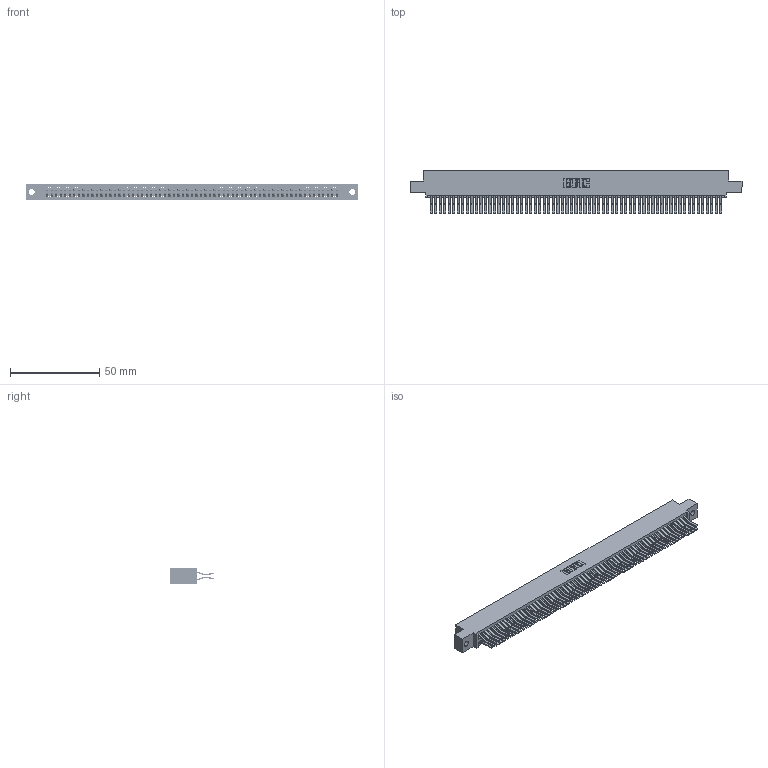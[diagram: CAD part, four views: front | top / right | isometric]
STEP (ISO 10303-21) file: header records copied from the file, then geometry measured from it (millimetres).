
FILE_DESCRIPTION (( 'STEP AP203' ), '1' );
FILE_NAME ('345-130-560-502.STEP', '2018-10-20T02:38:00', ( '' ), ( '' ), 'SwSTEP 2.0', 'SolidWorks 2016', '' );
FILE_SCHEMA (( 'CONFIG_CONTROL_DESIGN' ));
Length unit declared in the file: inch
Products named in the file (3): 345-292-001_560 Tail; 345 Part_0.110 Offset - 0.128 Dia; 345-130-560-502
Assembly tree (131 placements, depth 2):
  345-130-560-502
    345 Part_0.110 Offset - 0.128 Dia
    345-292-001_560 Tail  x130
Bounding box: 186.31 x 24.45 x 9.4 mm (x, y, z)
Volume: 19053.8 mm3; surface area: 30621.8 mm2
Topology: 131 solids, 131 shells, 6890 faces, 20503 edges, 13494 vertices
Faces by surface type: plane 4374, cylinder 2516
Entity records: 48127 total; most frequent: CARTESIAN_POINT 8048, ORIENTED_EDGE 7982, DIRECTION 7071, EDGE_CURVE 3991, VECTOR 3595, LINE 3595, VERTEX_POINT 2658, AXIS2_PLACEMENT_3D 1738
